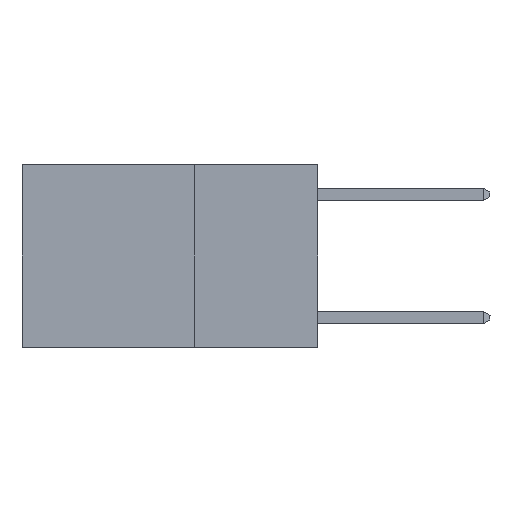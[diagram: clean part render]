
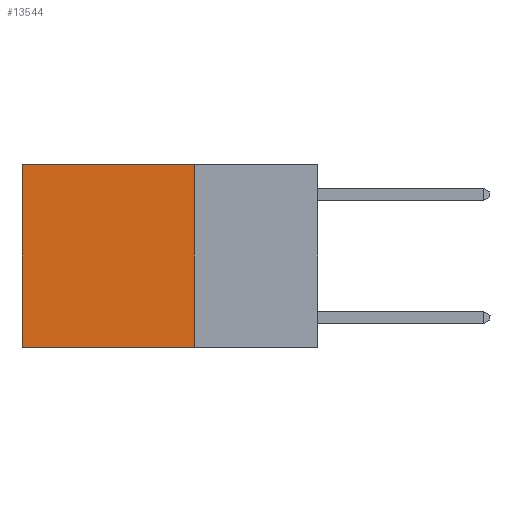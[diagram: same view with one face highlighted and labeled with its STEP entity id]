
A CAD part, left-side view. The second image highlights one B-rep face of the part: STEP entity #13544.
In plain terms, the highlighted planar face has unit normal (-1, 0, 0).
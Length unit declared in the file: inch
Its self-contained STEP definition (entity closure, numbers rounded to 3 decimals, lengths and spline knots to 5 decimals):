
#219 = CARTESIAN_POINT ( 'NONE',  ( 0.2625, 0.25, 0. ) ) ;
#311 = ORIENTED_EDGE ( 'NONE', *, *, #14585, .T. ) ;
#1080 = LINE ( 'NONE', #6603, #5866 ) ;
#1142 = VECTOR ( 'NONE', #10469, 39.37008 ) ;
#1989 = DIRECTION ( 'NONE',  ( 0., 0., -1. ) ) ;
#2288 = VERTEX_POINT ( 'NONE', #2327 ) ;
#2327 = CARTESIAN_POINT ( 'NONE',  ( 0.2625, 0.25, 0. ) ) ;
#2881 = DIRECTION ( 'NONE',  ( 0., 1., 0. ) ) ;
#3031 = DIRECTION ( 'NONE',  ( 0., 1., 0. ) ) ;
#4282 = DIRECTION ( 'NONE',  ( 0., 0., -1. ) ) ;
#5866 = VECTOR ( 'NONE', #3031, 39.37008 ) ;
#6523 = ORIENTED_EDGE ( 'NONE', *, *, #13733, .T. ) ;
#6603 = CARTESIAN_POINT ( 'NONE',  ( 0.2625, 0.25, -0.37 ) ) ;
#6912 = CARTESIAN_POINT ( 'NONE',  ( 0.2625, 0.25, 0. ) ) ;
#6994 = LINE ( 'NONE', #22201, #11123 ) ;
#7129 = CARTESIAN_POINT ( 'NONE',  ( 0.2625, 0.6, 0. ) ) ;
#7314 = VERTEX_POINT ( 'NONE', #10945 ) ;
#7351 = PLANE ( 'NONE',  #16312 ) ;
#8392 = VERTEX_POINT ( 'NONE', #7129 ) ;
#9719 = EDGE_CURVE ( 'NONE', #2288, #19737, #10094, .T. ) ;
#10080 = LINE ( 'NONE', #14843, #18848 ) ;
#10094 = LINE ( 'NONE', #6912, #1142 ) ;
#10469 = DIRECTION ( 'NONE',  ( 0., 0., -1. ) ) ;
#10945 = CARTESIAN_POINT ( 'NONE',  ( 0.2625, 0.6, -0.37 ) ) ;
#11123 = VECTOR ( 'NONE', #2881, 39.37008 ) ;
#12162 = ORIENTED_EDGE ( 'NONE', *, *, #9719, .F. ) ;
#12658 = DIRECTION ( 'NONE',  ( 1., 0., 0. ) ) ;
#13544 = ADVANCED_FACE ( 'NONE', ( #17498 ), #7351, .F. ) ;
#13733 = EDGE_CURVE ( 'NONE', #8392, #7314, #10080, .T. ) ;
#14585 = EDGE_CURVE ( 'NONE', #2288, #8392, #6994, .T. ) ;
#14618 = EDGE_CURVE ( 'NONE', #19737, #7314, #1080, .T. ) ;
#14843 = CARTESIAN_POINT ( 'NONE',  ( 0.2625, 0.6, 0. ) ) ;
#16312 = AXIS2_PLACEMENT_3D ( 'NONE', #219, #12658, #1989 ) ;
#16628 = EDGE_LOOP ( 'NONE', ( #6523, #17174, #12162, #311 ) ) ;
#17174 = ORIENTED_EDGE ( 'NONE', *, *, #14618, .F. ) ;
#17498 = FACE_OUTER_BOUND ( 'NONE', #16628, .T. ) ;
#18848 = VECTOR ( 'NONE', #4282, 39.37008 ) ;
#19737 = VERTEX_POINT ( 'NONE', #22783 ) ;
#22201 = CARTESIAN_POINT ( 'NONE',  ( 0.2625, 0.25, 0. ) ) ;
#22783 = CARTESIAN_POINT ( 'NONE',  ( 0.2625, 0.25, -0.37 ) ) ;
